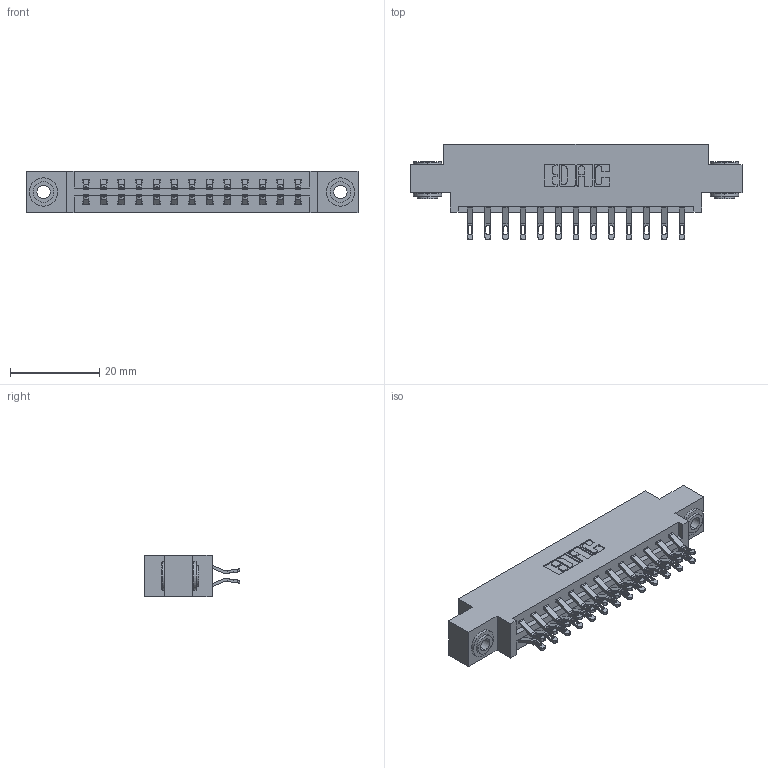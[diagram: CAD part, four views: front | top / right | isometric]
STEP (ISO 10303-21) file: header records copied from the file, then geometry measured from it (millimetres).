
FILE_DESCRIPTION (( 'STEP AP203' ), '1' );
FILE_NAME ('387-026-555-803.STEP', '2019-10-16T20:36:07', ( '' ), ( '' ), 'SwSTEP 2.0', 'SolidWorks 2016', '' );
FILE_SCHEMA (( 'CONFIG_CONTROL_DESIGN' ));
Length unit declared in the file: inch
Products named in the file (4): 345-250-002_345-250-002-102; 337 Part_0.170 Offset - 0.156 Dia-TH; 345-292-001_555 Tail; 387-026-555-803
Assembly tree (29 placements, depth 2):
  387-026-555-803
    337 Part_0.170 Offset - 0.156 Dia-TH
    345-292-001_555 Tail  x26
    345-250-002_345-250-002-102  x2
Bounding box: 74.52 x 21.47 x 9.4 mm (x, y, z)
Volume: 7445.2 mm3; surface area: 8751.5 mm2
Topology: 29 solids, 29 shells, 1716 faces, 5313 edges, 3538 vertices
Faces by surface type: plane 1020, cylinder 688, cone 8
Entity records: 14938 total; most frequent: CARTESIAN_POINT 2551, ORIENTED_EDGE 2450, DIRECTION 2227, EDGE_CURVE 1225, LINE 1053, VECTOR 1053, VERTEX_POINT 814, AXIS2_PLACEMENT_3D 587
